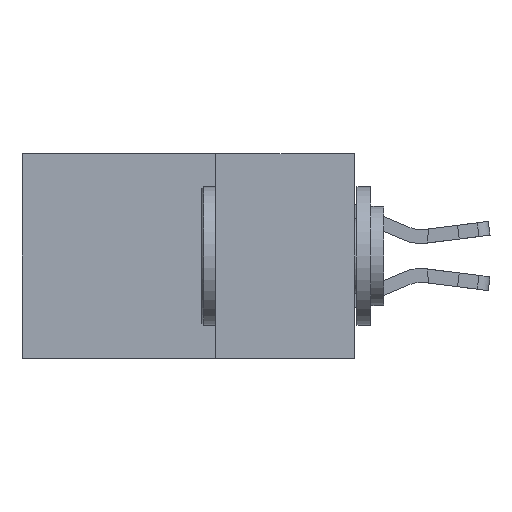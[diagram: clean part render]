
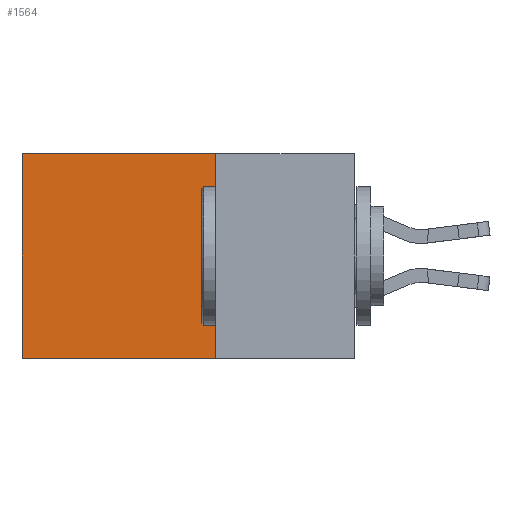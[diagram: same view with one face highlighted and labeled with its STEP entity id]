
A CAD part, left-side view. The second image highlights one B-rep face of the part: STEP entity #1564.
In plain terms, the highlighted planar face has unit normal (-1, 0, 0).
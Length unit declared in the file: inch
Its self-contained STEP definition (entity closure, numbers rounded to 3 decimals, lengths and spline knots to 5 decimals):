
#297 = CARTESIAN_POINT ( 'NONE',  ( 0.298, 0.6, 0. ) ) ;
#561 = LINE ( 'NONE', #19465, #17079 ) ;
#610 = LINE ( 'NONE', #297, #4533 ) ;
#693 = CARTESIAN_POINT ( 'NONE',  ( 0.298, 0.6, -0.37 ) ) ;
#1192 = EDGE_CURVE ( 'NONE', #19177, #8505, #561, .T. ) ;
#1488 = ORIENTED_EDGE ( 'NONE', *, *, #1192, .T. ) ;
#1564 = ADVANCED_FACE ( 'NONE', ( #14454 ), #18560, .F. ) ;
#1998 = DIRECTION ( 'NONE',  ( 0., 0., -1. ) ) ;
#2205 = VERTEX_POINT ( 'NONE', #14184 ) ;
#2310 = ORIENTED_EDGE ( 'NONE', *, *, #8252, .T. ) ;
#2827 = CARTESIAN_POINT ( 'NONE',  ( 0.298, 0.25, -0.37 ) ) ;
#3155 = EDGE_CURVE ( 'NONE', #19177, #2205, #8867, .T. ) ;
#4533 = VECTOR ( 'NONE', #1998, 39.37008 ) ;
#4827 = CARTESIAN_POINT ( 'NONE',  ( 0.298, 0.25, 0. ) ) ;
#5928 = VERTEX_POINT ( 'NONE', #693 ) ;
#8252 = EDGE_CURVE ( 'NONE', #8505, #5928, #610, .T. ) ;
#8505 = VERTEX_POINT ( 'NONE', #12331 ) ;
#8867 = LINE ( 'NONE', #19255, #9393 ) ;
#9393 = VECTOR ( 'NONE', #13664, 39.37008 ) ;
#9636 = EDGE_LOOP ( 'NONE', ( #2310, #12870, #16818, #1488 ) ) ;
#12331 = CARTESIAN_POINT ( 'NONE',  ( 0.298, 0.6, 0. ) ) ;
#12870 = ORIENTED_EDGE ( 'NONE', *, *, #18514, .F. ) ;
#13664 = DIRECTION ( 'NONE',  ( 0., 0., -1. ) ) ;
#14006 = VECTOR ( 'NONE', #17119, 39.37008 ) ;
#14184 = CARTESIAN_POINT ( 'NONE',  ( 0.298, 0.25, -0.37 ) ) ;
#14454 = FACE_OUTER_BOUND ( 'NONE', #9636, .T. ) ;
#14914 = AXIS2_PLACEMENT_3D ( 'NONE', #18471, #19272, #19250 ) ;
#16818 = ORIENTED_EDGE ( 'NONE', *, *, #3155, .F. ) ;
#17079 = VECTOR ( 'NONE', #20446, 39.37008 ) ;
#17106 = LINE ( 'NONE', #2827, #14006 ) ;
#17119 = DIRECTION ( 'NONE',  ( 0., 1., 0. ) ) ;
#18471 = CARTESIAN_POINT ( 'NONE',  ( 0.298, 0.25, 0. ) ) ;
#18514 = EDGE_CURVE ( 'NONE', #2205, #5928, #17106, .T. ) ;
#18560 = PLANE ( 'NONE',  #14914 ) ;
#19177 = VERTEX_POINT ( 'NONE', #4827 ) ;
#19250 = DIRECTION ( 'NONE',  ( 0., 0., -1. ) ) ;
#19255 = CARTESIAN_POINT ( 'NONE',  ( 0.298, 0.25, 0. ) ) ;
#19272 = DIRECTION ( 'NONE',  ( 1., 0., 0. ) ) ;
#19465 = CARTESIAN_POINT ( 'NONE',  ( 0.298, 0.25, 0. ) ) ;
#20446 = DIRECTION ( 'NONE',  ( 0., 1., 0. ) ) ;
